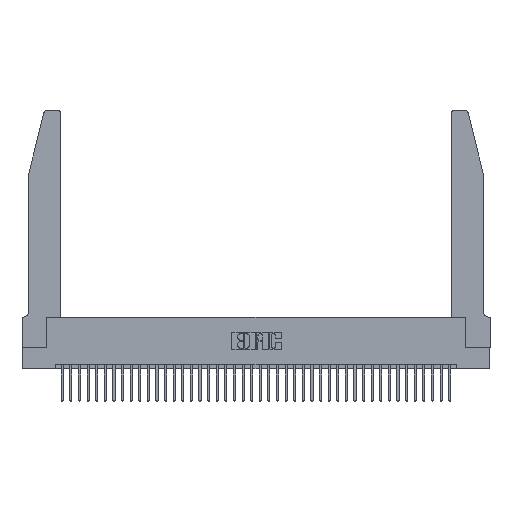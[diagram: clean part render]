
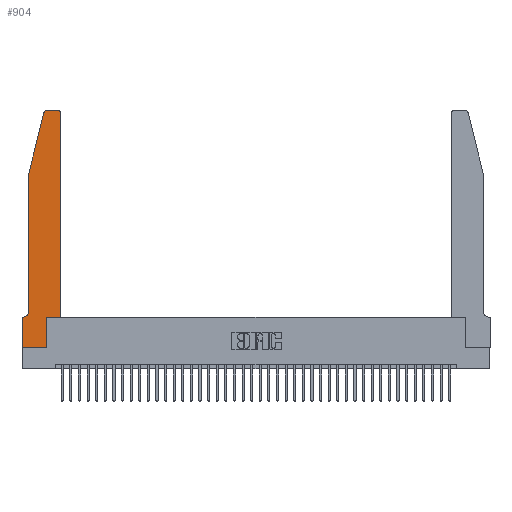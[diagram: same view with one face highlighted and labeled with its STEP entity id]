
A CAD part, top view. The second image highlights one B-rep face of the part: STEP entity #904.
In plain terms, the highlighted planar face has unit normal (0, 0, 1).
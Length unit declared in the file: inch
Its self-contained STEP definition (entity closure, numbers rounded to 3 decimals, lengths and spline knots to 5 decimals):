
#9 = VERTEX_POINT ( 'NONE', #26803 ) ;
#292 = EDGE_CURVE ( 'NONE', #10080, #3745, #10876, .T. ) ;
#326 = CARTESIAN_POINT ( 'NONE',  ( 0.4205, 2.72, 0.37 ) ) ;
#338 = DIRECTION ( 'NONE',  ( 1., 0., 0. ) ) ;
#656 = LINE ( 'NONE', #23679, #5068 ) ;
#904 = ADVANCED_FACE ( 'NONE', ( #3512 ), #33250, .T. ) ;
#1251 = DIRECTION ( 'NONE',  ( -1., 0., 0. ) ) ;
#1755 = CARTESIAN_POINT ( 'NONE',  ( 0.0055, 0.42, 0.37 ) ) ;
#2397 = VERTEX_POINT ( 'NONE', #31132 ) ;
#2600 = VECTOR ( 'NONE', #27290, 39.37008 ) ;
#2832 = CARTESIAN_POINT ( 'NONE',  ( 0., 0.35, 0.37 ) ) ;
#3384 = AXIS2_PLACEMENT_3D ( 'NONE', #1755, #20380, #7994 ) ;
#3512 = FACE_OUTER_BOUND ( 'NONE', #20835, .T. ) ;
#3745 = VERTEX_POINT ( 'NONE', #2832 ) ;
#4771 = VERTEX_POINT ( 'NONE', #10682 ) ;
#4923 = EDGE_CURVE ( 'NONE', #40004, #23131, #33923, .T. ) ;
#5068 = VECTOR ( 'NONE', #35695, 39.37008 ) ;
#5884 = VERTEX_POINT ( 'NONE', #25033 ) ;
#6475 = CARTESIAN_POINT ( 'NONE',  ( 0.4505, 0.35, 0.37 ) ) ;
#6781 = ORIENTED_EDGE ( 'NONE', *, *, #20838, .T. ) ;
#6785 = ORIENTED_EDGE ( 'NONE', *, *, #21329, .T. ) ;
#7855 = ORIENTED_EDGE ( 'NONE', *, *, #4923, .T. ) ;
#7986 = CARTESIAN_POINT ( 'NONE',  ( 0., 0., 0.37 ) ) ;
#7994 = DIRECTION ( 'NONE',  ( -1., 0., 0. ) ) ;
#8508 = CARTESIAN_POINT ( 'NONE',  ( 0.2865, 0.35, 0.37 ) ) ;
#9561 = EDGE_CURVE ( 'NONE', #2397, #5884, #26177, .T. ) ;
#9797 = DIRECTION ( 'NONE',  ( 1., 0., 0. ) ) ;
#10080 = VERTEX_POINT ( 'NONE', #31760 ) ;
#10576 = CIRCLE ( 'NONE', #20417, 0.03 ) ;
#10682 = CARTESIAN_POINT ( 'NONE',  ( 0.4505, 0.35, 0.37 ) ) ;
#10692 = DIRECTION ( 'NONE',  ( 1., 0., 0. ) ) ;
#10876 = LINE ( 'NONE', #24561, #2600 ) ;
#10957 = CARTESIAN_POINT ( 'NONE',  ( 0.2605, 2.75, 0.37 ) ) ;
#11600 = VECTOR ( 'NONE', #9797, 39.37008 ) ;
#11700 = DIRECTION ( 'NONE',  ( 0., 0., 1. ) ) ;
#11774 = DIRECTION ( 'NONE',  ( 1., 0., 0. ) ) ;
#11790 = ORIENTED_EDGE ( 'NONE', *, *, #32548, .T. ) ;
#12137 = CARTESIAN_POINT ( 'NONE',  ( 0., 0., 0.37 ) ) ;
#12942 = EDGE_CURVE ( 'NONE', #21469, #10080, #21621, .T. ) ;
#13226 = VECTOR ( 'NONE', #22829, 39.37008 ) ;
#13763 = LINE ( 'NONE', #8508, #13226 ) ;
#15012 = ORIENTED_EDGE ( 'NONE', *, *, #33836, .T. ) ;
#17352 = AXIS2_PLACEMENT_3D ( 'NONE', #39660, #11700, #26852 ) ;
#17542 = EDGE_CURVE ( 'NONE', #5884, #40004, #10576, .T. ) ;
#17769 = CARTESIAN_POINT ( 'NONE',  ( 0.0755, 0.42, 0.37 ) ) ;
#17987 = AXIS2_PLACEMENT_3D ( 'NONE', #326, #27898, #10692 ) ;
#18553 = CARTESIAN_POINT ( 'NONE',  ( 0.25487, 2.72718, 0.37 ) ) ;
#18572 = CARTESIAN_POINT ( 'NONE',  ( 0.284, 2.72, 0.37 ) ) ;
#18618 = EDGE_CURVE ( 'NONE', #3745, #36853, #29808, .T. ) ;
#19823 = DIRECTION ( 'NONE',  ( 0., -1., 0. ) ) ;
#20108 = LINE ( 'NONE', #6475, #39144 ) ;
#20380 = DIRECTION ( 'NONE',  ( 0., 0., -1. ) ) ;
#20417 = AXIS2_PLACEMENT_3D ( 'NONE', #18572, #36856, #11774 ) ;
#20768 = LINE ( 'NONE', #23081, #24185 ) ;
#20835 = EDGE_LOOP ( 'NONE', ( #25321, #21710, #7855, #11790, #32199, #21194, #36638, #33159, #6785, #6781, #15012, #33232 ) ) ;
#20838 = EDGE_CURVE ( 'NONE', #9, #4771, #20108, .T. ) ;
#21075 = CARTESIAN_POINT ( 'NONE',  ( 0.2865, 0., 0.37 ) ) ;
#21194 = ORIENTED_EDGE ( 'NONE', *, *, #292, .T. ) ;
#21329 = EDGE_CURVE ( 'NONE', #31897, #9, #13763, .T. ) ;
#21469 = VERTEX_POINT ( 'NONE', #17769 ) ;
#21621 = CIRCLE ( 'NONE', #3384, 0.07 ) ;
#21710 = ORIENTED_EDGE ( 'NONE', *, *, #17542, .T. ) ;
#21821 = LINE ( 'NONE', #12137, #11600 ) ;
#22303 = CARTESIAN_POINT ( 'NONE',  ( 0., 0., 0.37 ) ) ;
#22829 = DIRECTION ( 'NONE',  ( 0., 1., 0. ) ) ;
#22931 = CARTESIAN_POINT ( 'NONE',  ( 0.4505, 2.72, 0.37 ) ) ;
#23081 = CARTESIAN_POINT ( 'NONE',  ( 0.0755, 2., 0.37 ) ) ;
#23131 = VERTEX_POINT ( 'NONE', #23188 ) ;
#23188 = CARTESIAN_POINT ( 'NONE',  ( 0.0755, 2., 0.37 ) ) ;
#23656 = VECTOR ( 'NONE', #26979, 39.37008 ) ;
#23679 = CARTESIAN_POINT ( 'NONE',  ( 0.4505, 0.35, 0.37 ) ) ;
#24185 = VECTOR ( 'NONE', #19823, 39.37008 ) ;
#24561 = CARTESIAN_POINT ( 'NONE',  ( 0.0755, 0.35, 0.37 ) ) ;
#25033 = CARTESIAN_POINT ( 'NONE',  ( 0.284, 2.75, 0.37 ) ) ;
#25321 = ORIENTED_EDGE ( 'NONE', *, *, #9561, .T. ) ;
#25732 = DIRECTION ( 'NONE',  ( 0., -1., 0. ) ) ;
#26177 = LINE ( 'NONE', #10957, #27185 ) ;
#26803 = CARTESIAN_POINT ( 'NONE',  ( 0.2865, 0.35, 0.37 ) ) ;
#26852 = DIRECTION ( 'NONE',  ( 1., 0., 0. ) ) ;
#26979 = DIRECTION ( 'NONE',  ( -0.239, -0.971, 0. ) ) ;
#27185 = VECTOR ( 'NONE', #1251, 39.37008 ) ;
#27290 = DIRECTION ( 'NONE',  ( -1., 0., 0. ) ) ;
#27898 = DIRECTION ( 'NONE',  ( 0., 0., 1. ) ) ;
#28407 = CIRCLE ( 'NONE', #17987, 0.03 ) ;
#28529 = VERTEX_POINT ( 'NONE', #22931 ) ;
#29808 = LINE ( 'NONE', #22303, #34684 ) ;
#31132 = CARTESIAN_POINT ( 'NONE',  ( 0.4205, 2.75, 0.37 ) ) ;
#31476 = EDGE_CURVE ( 'NONE', #36853, #31897, #21821, .T. ) ;
#31760 = CARTESIAN_POINT ( 'NONE',  ( 0.0055, 0.35, 0.37 ) ) ;
#31897 = VERTEX_POINT ( 'NONE', #21075 ) ;
#32199 = ORIENTED_EDGE ( 'NONE', *, *, #12942, .T. ) ;
#32548 = EDGE_CURVE ( 'NONE', #23131, #21469, #20768, .T. ) ;
#33120 = CARTESIAN_POINT ( 'NONE',  ( 0.0755, 2., 0.37 ) ) ;
#33159 = ORIENTED_EDGE ( 'NONE', *, *, #31476, .T. ) ;
#33232 = ORIENTED_EDGE ( 'NONE', *, *, #35167, .T. ) ;
#33250 = PLANE ( 'NONE',  #17352 ) ;
#33836 = EDGE_CURVE ( 'NONE', #4771, #28529, #656, .T. ) ;
#33923 = LINE ( 'NONE', #33120, #23656 ) ;
#34684 = VECTOR ( 'NONE', #25732, 39.37008 ) ;
#35167 = EDGE_CURVE ( 'NONE', #28529, #2397, #28407, .T. ) ;
#35695 = DIRECTION ( 'NONE',  ( 0., 1., 0. ) ) ;
#36638 = ORIENTED_EDGE ( 'NONE', *, *, #18618, .T. ) ;
#36853 = VERTEX_POINT ( 'NONE', #7986 ) ;
#36856 = DIRECTION ( 'NONE',  ( 0., 0., 1. ) ) ;
#39144 = VECTOR ( 'NONE', #338, 39.37008 ) ;
#39660 = CARTESIAN_POINT ( 'NONE',  ( 0., 0.35, 0.37 ) ) ;
#40004 = VERTEX_POINT ( 'NONE', #18553 ) ;
